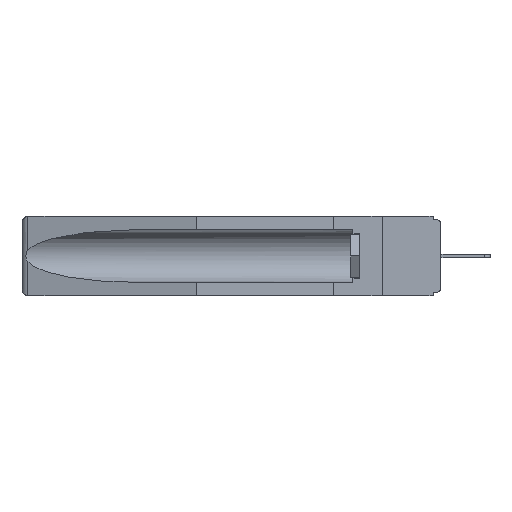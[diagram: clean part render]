
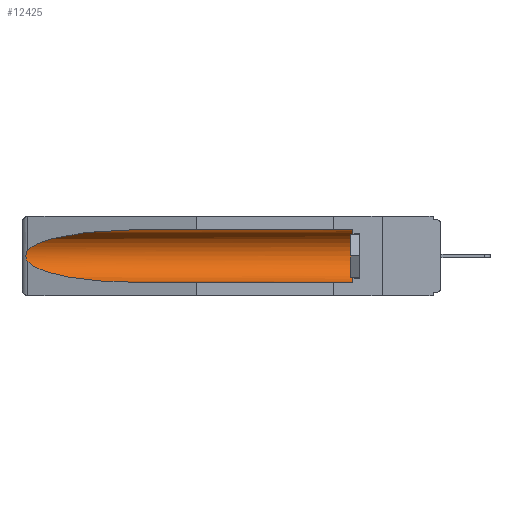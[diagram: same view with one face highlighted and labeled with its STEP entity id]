
A CAD part, left-side view. The second image highlights one B-rep face of the part: STEP entity #12425.
In plain terms, the highlighted cylindrical face has radius 2.857 mm (diameter 5.715 mm), a partial arc.
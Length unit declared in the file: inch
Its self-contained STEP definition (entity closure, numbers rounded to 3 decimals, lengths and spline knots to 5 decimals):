
#965 = CARTESIAN_POINT ( 'NONE',  ( 0.26537, 1.52718, -0.14972 ) ) ;
#1367 = CARTESIAN_POINT ( 'NONE',  ( 0.155, 1.07973, -0.284 ) ) ;
#1584 = ORIENTED_EDGE ( 'NONE', *, *, #5925, .F. ) ;
#1696 = ORIENTED_EDGE ( 'NONE', *, *, #11457, .T. ) ;
#1726 = CARTESIAN_POINT ( 'NONE',  ( 0.155, -0.30754, -0.059 ) ) ;
#1772 =( BOUNDED_CURVE ( )  B_SPLINE_CURVE ( 3, ( #12307, #18444, #18921, #8052 ),
 .UNSPECIFIED., .F., .F. ) 
 B_SPLINE_CURVE_WITH_KNOTS ( ( 4, 4 ),
 ( 0.1948, 1.5708 ),
 .UNSPECIFIED. ) 
 CURVE ( )  GEOMETRIC_REPRESENTATION_ITEM ( )  RATIONAL_B_SPLINE_CURVE ( ( 1., 0.848, 0.848, 1. ) ) 
 REPRESENTATION_ITEM ( '' )  );
#3885 = CARTESIAN_POINT ( 'NONE',  ( 0.155, 1.07973, -0.059 ) ) ;
#4063 = CARTESIAN_POINT ( 'NONE',  ( 0.26537, 1.52718, -0.14972 ) ) ;
#4453 = CARTESIAN_POINT ( 'NONE',  ( 0.155, 0.126, -0.1715 ) ) ;
#4503 = CARTESIAN_POINT ( 'NONE',  ( 0.155, -0.30754, -0.1715 ) ) ;
#4548 = CARTESIAN_POINT ( 'NONE',  ( 0.155, -0.30754, -0.284 ) ) ;
#4600 = VERTEX_POINT ( 'NONE', #13936 ) ;
#5097 = VECTOR ( 'NONE', #9375, 39.37008 ) ;
#5396 = CARTESIAN_POINT ( 'NONE',  ( 0.25451, 1.48313, -0.09465 ) ) ;
#5925 = EDGE_CURVE ( 'NONE', #17287, #17409, #6258, .T. ) ;
#6202 = CARTESIAN_POINT ( 'NONE',  ( 0.26655, 1.53094, -0.18657 ) ) ;
#6219 = DIRECTION ( 'NONE',  ( 0., 1., 0. ) ) ;
#6258 = LINE ( 'NONE', #4548, #16751 ) ;
#6655 = B_SPLINE_CURVE_WITH_KNOTS ( 'NONE', 3,
 ( #11944, #18075, #8918, #15049, #11032, #18583, #17168, #6202, #10841, #17064 ),
 .UNSPECIFIED., .F., .F.,
 ( 4, 2, 2, 2, 4 ),
 ( 0., 0.00029, 0.00058, 0.00087, 0.00117 ),
 .UNSPECIFIED. ) ;
#7121 = EDGE_LOOP ( 'NONE', ( #10527, #9313, #9677, #1584, #1696, #7957 ) ) ;
#7629 = CYLINDRICAL_SURFACE ( 'NONE', #17818, 0.1125 ) ;
#7770 = DIRECTION ( 'NONE',  ( 0., 1., 0. ) ) ;
#7957 = ORIENTED_EDGE ( 'NONE', *, *, #15353, .T. ) ;
#8048 =( BOUNDED_CURVE ( )  B_SPLINE_CURVE ( 3, ( #3885, #16252, #5396, #965 ),
 .UNSPECIFIED., .F., .F. ) 
 B_SPLINE_CURVE_WITH_KNOTS ( ( 4, 4 ),
 ( 4.71239, 6.08839 ),
 .UNSPECIFIED. ) 
 CURVE ( )  GEOMETRIC_REPRESENTATION_ITEM ( )  RATIONAL_B_SPLINE_CURVE ( ( 1., 0.848, 0.848, 1. ) ) 
 REPRESENTATION_ITEM ( '' )  );
#8052 = CARTESIAN_POINT ( 'NONE',  ( 0.155, 1.07973, -0.284 ) ) ;
#8329 = CARTESIAN_POINT ( 'NONE',  ( 0.155, 0.126, -0.284 ) ) ;
#8918 = CARTESIAN_POINT ( 'NONE',  ( 0.26654, 1.53092, -0.15636 ) ) ;
#9313 = ORIENTED_EDGE ( 'NONE', *, *, #14432, .T. ) ;
#9375 = DIRECTION ( 'NONE',  ( 0., 1., 0. ) ) ;
#9677 = ORIENTED_EDGE ( 'NONE', *, *, #19558, .T. ) ;
#10030 = CARTESIAN_POINT ( 'NONE',  ( 0.155, 1.07973, -0.059 ) ) ;
#10201 = DIRECTION ( 'NONE',  ( 0., 0., 1. ) ) ;
#10527 = ORIENTED_EDGE ( 'NONE', *, *, #10953, .T. ) ;
#10650 = DIRECTION ( 'NONE',  ( 0., 0., 1. ) ) ;
#10841 = CARTESIAN_POINT ( 'NONE',  ( 0.26597, 1.5296, -0.19026 ) ) ;
#10953 = EDGE_CURVE ( 'NONE', #14176, #11468, #8048, .T. ) ;
#11032 = CARTESIAN_POINT ( 'NONE',  ( 0.2675, 1.53308, -0.16763 ) ) ;
#11457 = EDGE_CURVE ( 'NONE', #17287, #4600, #19132, .T. ) ;
#11468 = VERTEX_POINT ( 'NONE', #4063 ) ;
#11742 = AXIS2_PLACEMENT_3D ( 'NONE', #4453, #17937, #10201 ) ;
#11944 = CARTESIAN_POINT ( 'NONE',  ( 0.26537, 1.52718, -0.14972 ) ) ;
#12195 = LINE ( 'NONE', #1726, #5097 ) ;
#12307 = CARTESIAN_POINT ( 'NONE',  ( 0.26537, 1.52718, -0.19328 ) ) ;
#12425 = ADVANCED_FACE ( 'NONE', ( #15366 ), #7629, .F. ) ;
#13806 = VERTEX_POINT ( 'NONE', #14205 ) ;
#13936 = CARTESIAN_POINT ( 'NONE',  ( 0.155, 0.126, -0.059 ) ) ;
#14176 = VERTEX_POINT ( 'NONE', #10030 ) ;
#14205 = CARTESIAN_POINT ( 'NONE',  ( 0.26537, 1.52718, -0.19328 ) ) ;
#14432 = EDGE_CURVE ( 'NONE', #11468, #13806, #6655, .T. ) ;
#15049 = CARTESIAN_POINT ( 'NONE',  ( 0.2673, 1.5327, -0.16383 ) ) ;
#15353 = EDGE_CURVE ( 'NONE', #4600, #14176, #12195, .T. ) ;
#15366 = FACE_OUTER_BOUND ( 'NONE', #7121, .T. ) ;
#16252 = CARTESIAN_POINT ( 'NONE',  ( 0.21114, 1.30732, -0.059 ) ) ;
#16751 = VECTOR ( 'NONE', #7770, 39.37008 ) ;
#17064 = CARTESIAN_POINT ( 'NONE',  ( 0.26537, 1.52718, -0.19328 ) ) ;
#17168 = CARTESIAN_POINT ( 'NONE',  ( 0.2673, 1.53269, -0.17917 ) ) ;
#17287 = VERTEX_POINT ( 'NONE', #8329 ) ;
#17409 = VERTEX_POINT ( 'NONE', #1367 ) ;
#17818 = AXIS2_PLACEMENT_3D ( 'NONE', #4503, #6219, #10650 ) ;
#17937 = DIRECTION ( 'NONE',  ( 0., -1., 0. ) ) ;
#18075 = CARTESIAN_POINT ( 'NONE',  ( 0.26597, 1.52961, -0.15275 ) ) ;
#18444 = CARTESIAN_POINT ( 'NONE',  ( 0.25451, 1.48313, -0.24835 ) ) ;
#18583 = CARTESIAN_POINT ( 'NONE',  ( 0.2675, 1.53308, -0.17534 ) ) ;
#18921 = CARTESIAN_POINT ( 'NONE',  ( 0.21114, 1.30732, -0.284 ) ) ;
#19132 = CIRCLE ( 'NONE', #11742, 0.1125 ) ;
#19558 = EDGE_CURVE ( 'NONE', #13806, #17409, #1772, .T. ) ;
